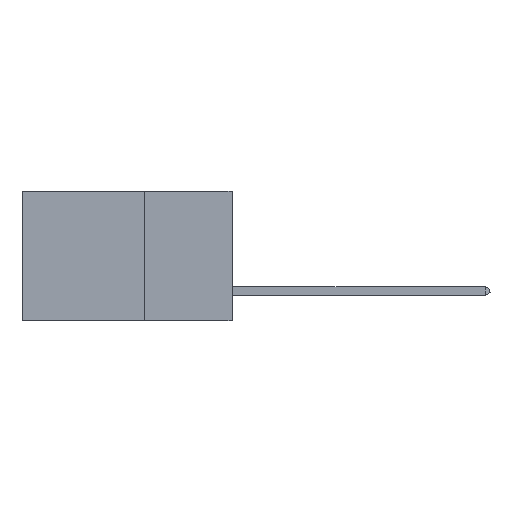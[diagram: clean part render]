
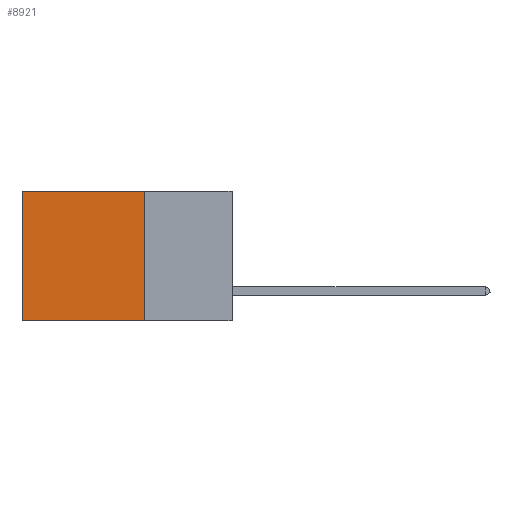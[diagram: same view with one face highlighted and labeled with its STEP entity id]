
A CAD part, left-side view. The second image highlights one B-rep face of the part: STEP entity #8921.
In plain terms, the highlighted planar face has unit normal (-1, 0, 0).
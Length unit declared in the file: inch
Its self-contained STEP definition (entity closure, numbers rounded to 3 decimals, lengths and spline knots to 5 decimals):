
#100 = EDGE_CURVE ( 'NONE', #9435, #15795, #5662, .T. ) ;
#365 = CARTESIAN_POINT ( 'NONE',  ( 0.2875, 0.25, -0.37 ) ) ;
#458 = FACE_OUTER_BOUND ( 'NONE', #5935, .T. ) ;
#612 = CARTESIAN_POINT ( 'NONE',  ( 0.2875, 0.6, 0. ) ) ;
#1200 = AXIS2_PLACEMENT_3D ( 'NONE', #14530, #6123, #4695 ) ;
#1562 = EDGE_CURVE ( 'NONE', #7429, #9435, #10753, .T. ) ;
#1797 = DIRECTION ( 'NONE',  ( 0., 1., 0. ) ) ;
#2264 = VECTOR ( 'NONE', #5610, 39.37008 ) ;
#2302 = VECTOR ( 'NONE', #13187, 39.37008 ) ;
#3153 = VECTOR ( 'NONE', #1797, 39.37008 ) ;
#3930 = CARTESIAN_POINT ( 'NONE',  ( 0.2875, 0.25, 0. ) ) ;
#4695 = DIRECTION ( 'NONE',  ( 0., 0., -1. ) ) ;
#5610 = DIRECTION ( 'NONE',  ( 0., 0., -1. ) ) ;
#5662 = LINE ( 'NONE', #365, #3153 ) ;
#5910 = CARTESIAN_POINT ( 'NONE',  ( 0.2875, 0.25, 0. ) ) ;
#5935 = EDGE_LOOP ( 'NONE', ( #10052, #8541, #11385, #5963 ) ) ;
#5963 = ORIENTED_EDGE ( 'NONE', *, *, #12250, .T. ) ;
#6123 = DIRECTION ( 'NONE',  ( 1., 0., 0. ) ) ;
#6556 = LINE ( 'NONE', #5910, #2302 ) ;
#7429 = VERTEX_POINT ( 'NONE', #3930 ) ;
#8541 = ORIENTED_EDGE ( 'NONE', *, *, #100, .F. ) ;
#8578 = CARTESIAN_POINT ( 'NONE',  ( 0.2875, 0.6, -0.37 ) ) ;
#8921 = ADVANCED_FACE ( 'NONE', ( #458 ), #12070, .F. ) ;
#9435 = VERTEX_POINT ( 'NONE', #15569 ) ;
#9663 = VERTEX_POINT ( 'NONE', #10860 ) ;
#10052 = ORIENTED_EDGE ( 'NONE', *, *, #11716, .T. ) ;
#10391 = DIRECTION ( 'NONE',  ( 0., 0., -1. ) ) ;
#10753 = LINE ( 'NONE', #11684, #2264 ) ;
#10860 = CARTESIAN_POINT ( 'NONE',  ( 0.2875, 0.6, 0. ) ) ;
#11385 = ORIENTED_EDGE ( 'NONE', *, *, #1562, .F. ) ;
#11684 = CARTESIAN_POINT ( 'NONE',  ( 0.2875, 0.25, 0. ) ) ;
#11716 = EDGE_CURVE ( 'NONE', #9663, #15795, #14815, .T. ) ;
#11741 = VECTOR ( 'NONE', #10391, 39.37008 ) ;
#12070 = PLANE ( 'NONE',  #1200 ) ;
#12250 = EDGE_CURVE ( 'NONE', #7429, #9663, #6556, .T. ) ;
#13187 = DIRECTION ( 'NONE',  ( 0., 1., 0. ) ) ;
#14530 = CARTESIAN_POINT ( 'NONE',  ( 0.2875, 0.25, 0. ) ) ;
#14815 = LINE ( 'NONE', #612, #11741 ) ;
#15569 = CARTESIAN_POINT ( 'NONE',  ( 0.2875, 0.25, -0.37 ) ) ;
#15795 = VERTEX_POINT ( 'NONE', #8578 ) ;
